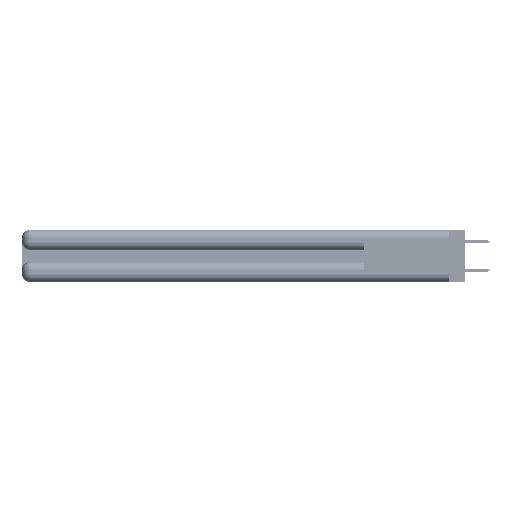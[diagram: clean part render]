
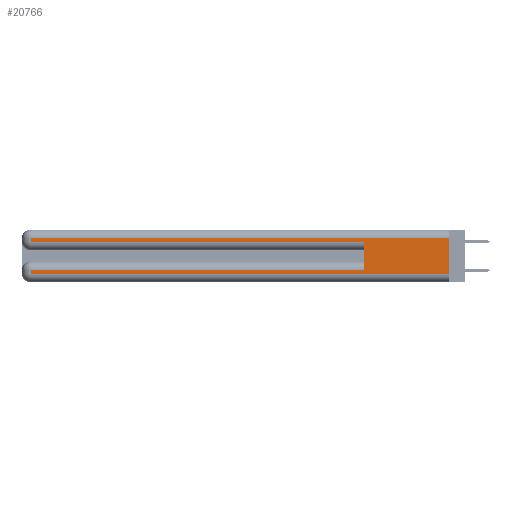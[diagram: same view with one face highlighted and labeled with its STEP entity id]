
A CAD part, left-side view. The second image highlights one B-rep face of the part: STEP entity #20766.
In plain terms, the highlighted planar face has unit normal (-1, 0, 0).
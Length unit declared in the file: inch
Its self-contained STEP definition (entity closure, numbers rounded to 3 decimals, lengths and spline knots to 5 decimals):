
#387 = CARTESIAN_POINT ( 'NONE',  ( 0., 2.94, 0.37 ) ) ;
#870 = CARTESIAN_POINT ( 'NONE',  ( 0., 0., 0.085 ) ) ;
#3162 = VECTOR ( 'NONE', #13114, 39.37008 ) ;
#4278 = ORIENTED_EDGE ( 'NONE', *, *, #12566, .F. ) ;
#4423 = LINE ( 'NONE', #15649, #12355 ) ;
#5063 = DIRECTION ( 'NONE',  ( 0., -1., 0. ) ) ;
#5934 = DIRECTION ( 'NONE',  ( 0., 0., -1. ) ) ;
#5978 = FACE_OUTER_BOUND ( 'NONE', #46750, .T. ) ;
#6041 = EDGE_CURVE ( 'NONE', #20153, #21383, #45763, .T. ) ;
#6864 = LINE ( 'NONE', #17772, #35324 ) ;
#7017 = LINE ( 'NONE', #41952, #27650 ) ;
#7235 = CARTESIAN_POINT ( 'NONE',  ( 0., 2.94, 0.31 ) ) ;
#7750 = CARTESIAN_POINT ( 'NONE',  ( 0., 2.94, 0.37 ) ) ;
#8874 = DIRECTION ( 'NONE',  ( 0., 1., 0. ) ) ;
#9484 = ORIENTED_EDGE ( 'NONE', *, *, #24273, .T. ) ;
#9748 = VECTOR ( 'NONE', #23398, 39.37008 ) ;
#10981 = LINE ( 'NONE', #7750, #9748 ) ;
#11848 = CARTESIAN_POINT ( 'NONE',  ( 0., 0., 0.06 ) ) ;
#12241 = VERTEX_POINT ( 'NONE', #40124 ) ;
#12329 = CARTESIAN_POINT ( 'NONE',  ( 0., 0., 0.31 ) ) ;
#12355 = VECTOR ( 'NONE', #31159, 39.37008 ) ;
#12566 = EDGE_CURVE ( 'NONE', #17475, #21383, #7017, .T. ) ;
#13114 = DIRECTION ( 'NONE',  ( 0., -1., 0. ) ) ;
#13647 = PLANE ( 'NONE',  #40788 ) ;
#13787 = VECTOR ( 'NONE', #5063, 39.37008 ) ;
#14463 = VERTEX_POINT ( 'NONE', #29904 ) ;
#15649 = CARTESIAN_POINT ( 'NONE',  ( 0., 0., 0.31 ) ) ;
#15809 = VERTEX_POINT ( 'NONE', #11848 ) ;
#16883 = CARTESIAN_POINT ( 'NONE',  ( 0., 0., 0.285 ) ) ;
#16949 = CARTESIAN_POINT ( 'NONE',  ( 0., 0.6, 0.085 ) ) ;
#17475 = VERTEX_POINT ( 'NONE', #16949 ) ;
#17578 = EDGE_CURVE ( 'NONE', #44462, #15809, #6864, .T. ) ;
#17772 = CARTESIAN_POINT ( 'NONE',  ( 0., 0., 0.37 ) ) ;
#18079 = EDGE_CURVE ( 'NONE', #12241, #15809, #23821, .T. ) ;
#18872 = DIRECTION ( 'NONE',  ( 0., 0., 1. ) ) ;
#20153 = VERTEX_POINT ( 'NONE', #41205 ) ;
#20766 = ADVANCED_FACE ( 'NONE', ( #5978 ), #13647, .F. ) ;
#21262 = CARTESIAN_POINT ( 'NONE',  ( 0., 0., 0.37 ) ) ;
#21383 = VERTEX_POINT ( 'NONE', #41278 ) ;
#21508 = VERTEX_POINT ( 'NONE', #7235 ) ;
#23398 = DIRECTION ( 'NONE',  ( 0., 0., -1. ) ) ;
#23821 = LINE ( 'NONE', #47654, #3162 ) ;
#24273 = EDGE_CURVE ( 'NONE', #21508, #20153, #38445, .T. ) ;
#27650 = VECTOR ( 'NONE', #18872, 39.37008 ) ;
#29184 = DIRECTION ( 'NONE',  ( 1., 0., 0. ) ) ;
#29404 = ORIENTED_EDGE ( 'NONE', *, *, #17578, .F. ) ;
#29904 = CARTESIAN_POINT ( 'NONE',  ( 0., 2.94, 0.085 ) ) ;
#30006 = VECTOR ( 'NONE', #8874, 39.37008 ) ;
#31159 = DIRECTION ( 'NONE',  ( 0., 1., 0. ) ) ;
#31442 = DIRECTION ( 'NONE',  ( 0., 0., -1. ) ) ;
#31633 = ORIENTED_EDGE ( 'NONE', *, *, #37195, .T. ) ;
#33661 = ORIENTED_EDGE ( 'NONE', *, *, #46529, .T. ) ;
#33974 = ORIENTED_EDGE ( 'NONE', *, *, #18079, .T. ) ;
#34247 = EDGE_CURVE ( 'NONE', #17475, #14463, #40261, .T. ) ;
#34334 = ORIENTED_EDGE ( 'NONE', *, *, #6041, .T. ) ;
#35324 = VECTOR ( 'NONE', #48864, 39.37008 ) ;
#37195 = EDGE_CURVE ( 'NONE', #14463, #12241, #10981, .T. ) ;
#38445 = LINE ( 'NONE', #387, #47419 ) ;
#40124 = CARTESIAN_POINT ( 'NONE',  ( 0., 2.94, 0.06 ) ) ;
#40261 = LINE ( 'NONE', #870, #30006 ) ;
#40788 = AXIS2_PLACEMENT_3D ( 'NONE', #21262, #29184, #5934 ) ;
#41205 = CARTESIAN_POINT ( 'NONE',  ( 0., 2.94, 0.285 ) ) ;
#41278 = CARTESIAN_POINT ( 'NONE',  ( 0., 0.6, 0.285 ) ) ;
#41952 = CARTESIAN_POINT ( 'NONE',  ( 0., 0.6, 0.145 ) ) ;
#44462 = VERTEX_POINT ( 'NONE', #12329 ) ;
#45763 = LINE ( 'NONE', #16883, #13787 ) ;
#46529 = EDGE_CURVE ( 'NONE', #44462, #21508, #4423, .T. ) ;
#46750 = EDGE_LOOP ( 'NONE', ( #29404, #33661, #9484, #34334, #4278, #47823, #31633, #33974 ) ) ;
#47419 = VECTOR ( 'NONE', #31442, 39.37008 ) ;
#47654 = CARTESIAN_POINT ( 'NONE',  ( 0., 0., 0.06 ) ) ;
#47823 = ORIENTED_EDGE ( 'NONE', *, *, #34247, .T. ) ;
#48864 = DIRECTION ( 'NONE',  ( 0., 0., -1. ) ) ;
